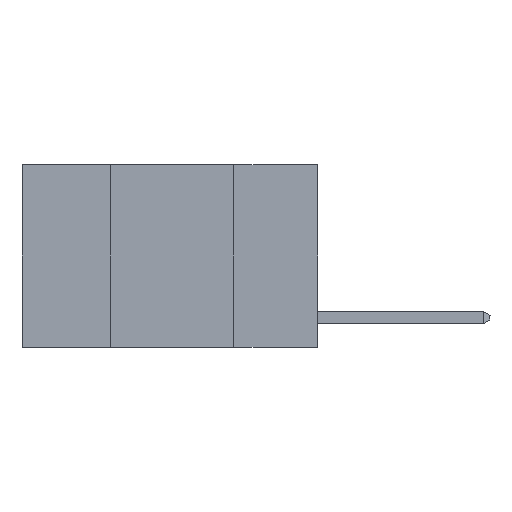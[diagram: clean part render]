
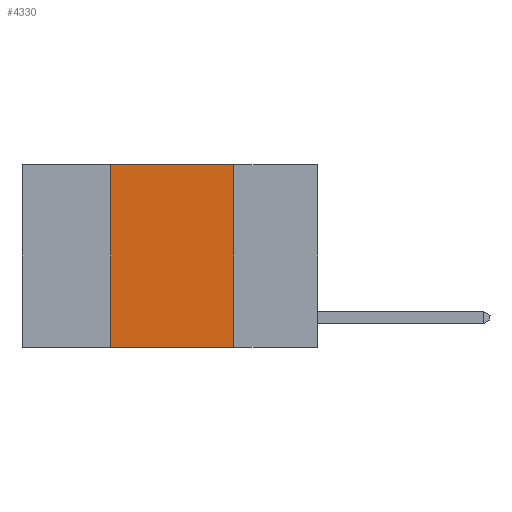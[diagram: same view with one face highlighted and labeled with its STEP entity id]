
A CAD part, left-side view. The second image highlights one B-rep face of the part: STEP entity #4330.
In plain terms, the highlighted planar face has unit normal (-1, 0, 0).
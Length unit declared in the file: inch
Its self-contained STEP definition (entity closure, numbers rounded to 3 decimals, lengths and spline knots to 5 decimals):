
#40 = CARTESIAN_POINT ( 'NONE',  ( 0., 0.6, 0. ) ) ;
#948 = CARTESIAN_POINT ( 'NONE',  ( 0., 0.42, 0. ) ) ;
#1260 = DIRECTION ( 'NONE',  ( 1., 0., 0. ) ) ;
#1350 = EDGE_CURVE ( 'NONE', #4421, #2724, #12255, .T. ) ;
#1512 = VERTEX_POINT ( 'NONE', #15663 ) ;
#2724 = VERTEX_POINT ( 'NONE', #16542 ) ;
#2757 = CARTESIAN_POINT ( 'NONE',  ( 0., 0.6, -0.37 ) ) ;
#2893 = DIRECTION ( 'NONE',  ( 0., -1., 0. ) ) ;
#2977 = DIRECTION ( 'NONE',  ( 0., 0., -1. ) ) ;
#4083 = DIRECTION ( 'NONE',  ( 0., 0., 1. ) ) ;
#4240 = ORIENTED_EDGE ( 'NONE', *, *, #12778, .F. ) ;
#4330 = ADVANCED_FACE ( 'NONE', ( #12171 ), #10833, .F. ) ;
#4421 = VERTEX_POINT ( 'NONE', #9792 ) ;
#7583 = CARTESIAN_POINT ( 'NONE',  ( 0., 0.6, 0. ) ) ;
#9099 = EDGE_CURVE ( 'NONE', #10432, #1512, #17313, .T. ) ;
#9171 = DIRECTION ( 'NONE',  ( 0., 0., -1. ) ) ;
#9792 = CARTESIAN_POINT ( 'NONE',  ( 0., 0.42, -0.37 ) ) ;
#10432 = VERTEX_POINT ( 'NONE', #17044 ) ;
#10833 = PLANE ( 'NONE',  #12793 ) ;
#11188 = VECTOR ( 'NONE', #11848, 39.37008 ) ;
#11848 = DIRECTION ( 'NONE',  ( 0., -1., 0. ) ) ;
#12171 = FACE_OUTER_BOUND ( 'NONE', #16424, .T. ) ;
#12255 = LINE ( 'NONE', #948, #16477 ) ;
#12778 = EDGE_CURVE ( 'NONE', #2724, #10432, #16865, .T. ) ;
#12793 = AXIS2_PLACEMENT_3D ( 'NONE', #40, #1260, #2977 ) ;
#13591 = VECTOR ( 'NONE', #9171, 39.37008 ) ;
#15377 = CARTESIAN_POINT ( 'NONE',  ( 0., 0.17, 0. ) ) ;
#15663 = CARTESIAN_POINT ( 'NONE',  ( 0., 0.17, -0.37 ) ) ;
#16424 = EDGE_LOOP ( 'NONE', ( #18963, #4240, #16437, #18816 ) ) ;
#16437 = ORIENTED_EDGE ( 'NONE', *, *, #1350, .F. ) ;
#16477 = VECTOR ( 'NONE', #4083, 39.37008 ) ;
#16542 = CARTESIAN_POINT ( 'NONE',  ( 0., 0.42, 0. ) ) ;
#16865 = LINE ( 'NONE', #7583, #17221 ) ;
#17044 = CARTESIAN_POINT ( 'NONE',  ( 0., 0.17, 0. ) ) ;
#17221 = VECTOR ( 'NONE', #2893, 39.37008 ) ;
#17313 = LINE ( 'NONE', #15377, #13591 ) ;
#18816 = ORIENTED_EDGE ( 'NONE', *, *, #19848, .T. ) ;
#18963 = ORIENTED_EDGE ( 'NONE', *, *, #9099, .F. ) ;
#19493 = LINE ( 'NONE', #2757, #11188 ) ;
#19848 = EDGE_CURVE ( 'NONE', #4421, #1512, #19493, .T. ) ;
